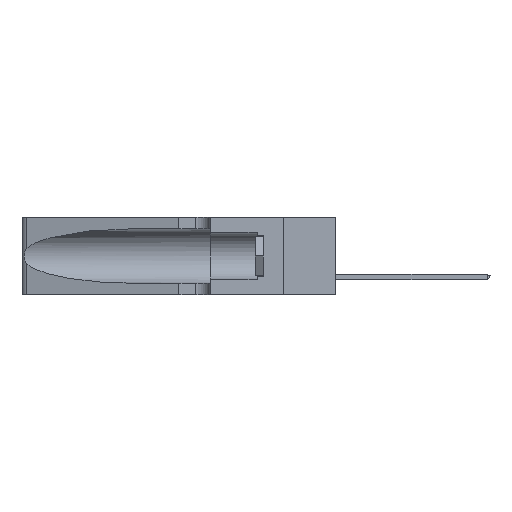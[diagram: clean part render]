
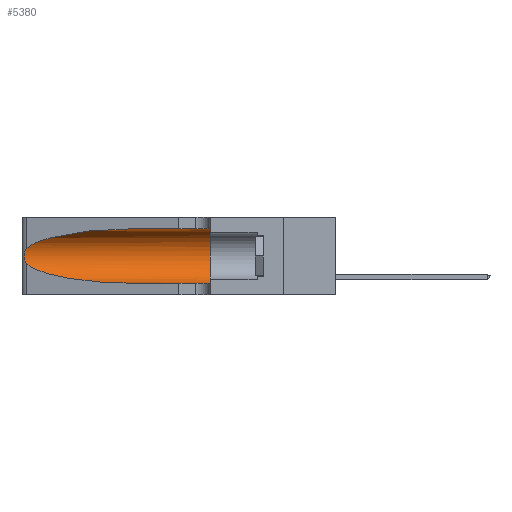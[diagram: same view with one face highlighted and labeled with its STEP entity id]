
A CAD part, left-side view. The second image highlights one B-rep face of the part: STEP entity #5380.
In plain terms, the highlighted cylindrical face has radius 3.308 mm (diameter 6.617 mm), a partial arc.
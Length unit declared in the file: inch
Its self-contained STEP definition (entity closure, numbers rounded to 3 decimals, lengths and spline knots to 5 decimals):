
#1091 = VERTEX_POINT ( 'NONE', #41570 ) ;
#1483 = CARTESIAN_POINT ( 'NONE',  ( 0.25787, 1.23484, 0.2124 ) ) ;
#2654 = VERTEX_POINT ( 'NONE', #5873 ) ;
#2913 = ORIENTED_EDGE ( 'NONE', *, *, #3441, .F. ) ;
#3441 = EDGE_CURVE ( 'NONE', #28787, #37115, #33061, .T. ) ;
#4282 = ORIENTED_EDGE ( 'NONE', *, *, #27592, .F. ) ;
#5134 = CARTESIAN_POINT ( 'NONE',  ( 0.25555, 1.22993, 0.14849 ) ) ;
#5380 = ADVANCED_FACE ( 'NONE', ( #21013 ), #17912, .F. ) ;
#5454 = DIRECTION ( 'NONE',  ( 0., 1., 0. ) ) ;
#5461 = CARTESIAN_POINT ( 'NONE',  ( 0.2373, 1.15595, 0.08982 ) ) ;
#5550 = VECTOR ( 'NONE', #20403, 39.37008 ) ;
#5725 = CARTESIAN_POINT ( 'NONE',  ( 0.25789, 1.23486, 0.15765 ) ) ;
#5873 = CARTESIAN_POINT ( 'NONE',  ( 0.25487, 1.22718, 0.22369 ) ) ;
#6259 = DIRECTION ( 'NONE',  ( 0., 0., -1. ) ) ;
#6381 = CARTESIAN_POINT ( 'NONE',  ( 0.25487, 1.22718, 0.14631 ) ) ;
#7022 = CARTESIAN_POINT ( 'NONE',  ( 0.25487, 1.22718, 0.14631 ) ) ;
#7099 = VERTEX_POINT ( 'NONE', #7022 ) ;
#7266 = CARTESIAN_POINT ( 'NONE',  ( 0.1305, 1.61858, 0.05475 ) ) ;
#7732 = CARTESIAN_POINT ( 'NONE',  ( 0.26075, 1.23896, 0.19203 ) ) ;
#8504 = CARTESIAN_POINT ( 'NONE',  ( 0.18966, 0.96281, 0.05475 ) ) ;
#9101 = CARTESIAN_POINT ( 'NONE',  ( 0.1305, 0.72297, 0.05475 ) ) ;
#11242 = CARTESIAN_POINT ( 'NONE',  ( 0.25555, 1.22994, 0.2215 ) ) ;
#11535 = CARTESIAN_POINT ( 'NONE',  ( 0.25854, 1.2359, 0.20912 ) ) ;
#11678 = CARTESIAN_POINT ( 'NONE',  ( 0.25487, 1.22718, 0.22369 ) ) ;
#12596 = EDGE_CURVE ( 'NONE', #18284, #37115, #40833, .T. ) ;
#15312 = CARTESIAN_POINT ( 'NONE',  ( 0.25856, 1.23593, 0.16098 ) ) ;
#16344 = LINE ( 'NONE', #24288, #22565 ) ;
#17912 = CYLINDRICAL_SURFACE ( 'NONE', #27255, 0.13025 ) ;
#18014 = EDGE_LOOP ( 'NONE', ( #30958, #41839, #38305, #20590, #2913, #4282 ) ) ;
#18284 = VERTEX_POINT ( 'NONE', #9101 ) ;
#18833 = CARTESIAN_POINT ( 'NONE',  ( 0.26075, 1.23896, 0.178 ) ) ;
#20278 = AXIS2_PLACEMENT_3D ( 'NONE', #32306, #5454, #41757 ) ;
#20368 = EDGE_CURVE ( 'NONE', #7099, #18284, #31611, .T. ) ;
#20403 = DIRECTION ( 'NONE',  ( 0., -1., 0. ) ) ;
#20590 = ORIENTED_EDGE ( 'NONE', *, *, #12596, .T. ) ;
#20650 = EDGE_CURVE ( 'NONE', #1091, #2654, #20709, .T. ) ;
#20709 =( BOUNDED_CURVE ( )  B_SPLINE_CURVE ( 3, ( #33392, #24007, #23729, #40487 ),
 .UNSPECIFIED., .F., .F. ) 
 B_SPLINE_CURVE_WITH_KNOTS ( ( 4, 4 ),
 ( 1.5708, 2.84003 ),
 .UNSPECIFIED. ) 
 CURVE ( )  GEOMETRIC_REPRESENTATION_ITEM ( )  RATIONAL_B_SPLINE_CURVE ( ( 1., 0.87, 0.87, 1. ) ) 
 REPRESENTATION_ITEM ( '' )  );
#21013 = FACE_OUTER_BOUND ( 'NONE', #18014, .T. ) ;
#21123 = CARTESIAN_POINT ( 'NONE',  ( 0.1305, 0.35, 0.05475 ) ) ;
#22565 = VECTOR ( 'NONE', #34680, 39.37008 ) ;
#23729 = CARTESIAN_POINT ( 'NONE',  ( 0.2373, 1.15595, 0.28018 ) ) ;
#23945 = EDGE_CURVE ( 'NONE', #2654, #7099, #29503, .T. ) ;
#24007 = CARTESIAN_POINT ( 'NONE',  ( 0.18966, 0.96281, 0.31525 ) ) ;
#24288 = CARTESIAN_POINT ( 'NONE',  ( 0.1305, 1.61858, 0.31525 ) ) ;
#27056 = DIRECTION ( 'NONE',  ( 0., -1., 0. ) ) ;
#27255 = AXIS2_PLACEMENT_3D ( 'NONE', #33976, #27056, #6259 ) ;
#27592 = EDGE_CURVE ( 'NONE', #1091, #28787, #16344, .T. ) ;
#28678 = CARTESIAN_POINT ( 'NONE',  ( 0.26017, 1.23833, 0.17102 ) ) ;
#28787 = VERTEX_POINT ( 'NONE', #39286 ) ;
#28958 = CARTESIAN_POINT ( 'NONE',  ( 0.25639, 1.23186, 0.15144 ) ) ;
#29503 = B_SPLINE_CURVE_WITH_KNOTS ( 'NONE', 3,
 ( #11678, #11242, #41291, #1483, #11535, #41458, #7732, #18833, #28678, #15312, #5725, #28958, #5134, #6381 ),
 .UNSPECIFIED., .F., .F.,
 ( 4, 2, 2, 2, 2, 2, 4 ),
 ( 0., 0.00027, 0.00053, 0.00107, 0.0016, 0.00187, 0.00214 ),
 .UNSPECIFIED. ) ;
#30958 = ORIENTED_EDGE ( 'NONE', *, *, #20650, .T. ) ;
#31611 =( BOUNDED_CURVE ( )  B_SPLINE_CURVE ( 3, ( #32311, #5461, #8504, #42908 ),
 .UNSPECIFIED., .F., .F. ) 
 B_SPLINE_CURVE_WITH_KNOTS ( ( 4, 4 ),
 ( 3.44316, 4.71239 ),
 .UNSPECIFIED. ) 
 CURVE ( )  GEOMETRIC_REPRESENTATION_ITEM ( )  RATIONAL_B_SPLINE_CURVE ( ( 1., 0.87, 0.87, 1. ) ) 
 REPRESENTATION_ITEM ( '' )  );
#32306 = CARTESIAN_POINT ( 'NONE',  ( 0.1305, 0.35, 0.185 ) ) ;
#32311 = CARTESIAN_POINT ( 'NONE',  ( 0.25487, 1.22718, 0.14631 ) ) ;
#33061 = CIRCLE ( 'NONE', #20278, 0.13025 ) ;
#33392 = CARTESIAN_POINT ( 'NONE',  ( 0.1305, 0.72297, 0.31525 ) ) ;
#33976 = CARTESIAN_POINT ( 'NONE',  ( 0.1305, 1.61858, 0.185 ) ) ;
#34680 = DIRECTION ( 'NONE',  ( 0., -1., 0. ) ) ;
#37115 = VERTEX_POINT ( 'NONE', #21123 ) ;
#38305 = ORIENTED_EDGE ( 'NONE', *, *, #20368, .T. ) ;
#39286 = CARTESIAN_POINT ( 'NONE',  ( 0.1305, 0.35, 0.31525 ) ) ;
#40487 = CARTESIAN_POINT ( 'NONE',  ( 0.25487, 1.22718, 0.22369 ) ) ;
#40833 = LINE ( 'NONE', #7266, #5550 ) ;
#41291 = CARTESIAN_POINT ( 'NONE',  ( 0.25639, 1.23184, 0.21858 ) ) ;
#41458 = CARTESIAN_POINT ( 'NONE',  ( 0.26018, 1.23835, 0.19895 ) ) ;
#41570 = CARTESIAN_POINT ( 'NONE',  ( 0.1305, 0.72297, 0.31525 ) ) ;
#41757 = DIRECTION ( 'NONE',  ( 0., 0., 1. ) ) ;
#41839 = ORIENTED_EDGE ( 'NONE', *, *, #23945, .T. ) ;
#42908 = CARTESIAN_POINT ( 'NONE',  ( 0.1305, 0.72297, 0.05475 ) ) ;
